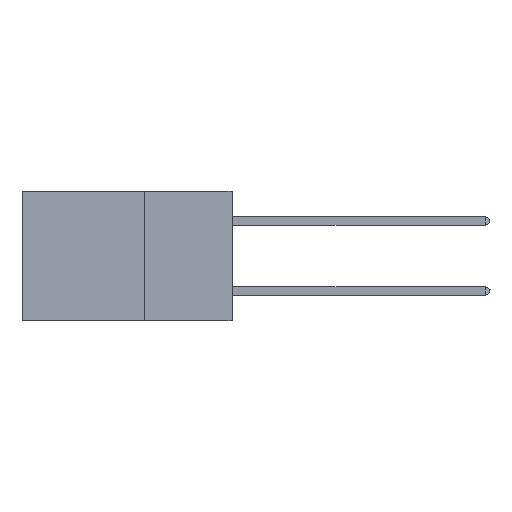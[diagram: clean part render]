
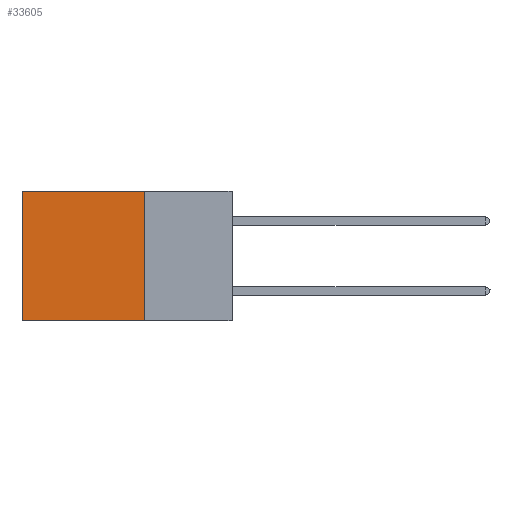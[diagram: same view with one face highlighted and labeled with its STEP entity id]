
A CAD part, left-side view. The second image highlights one B-rep face of the part: STEP entity #33605.
In plain terms, the highlighted planar face has unit normal (-1, 0, 0).
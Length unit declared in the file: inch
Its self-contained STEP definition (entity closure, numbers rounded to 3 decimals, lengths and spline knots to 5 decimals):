
#642 = CARTESIAN_POINT ( 'NONE',  ( 0.2875, 0.6, -0.37 ) ) ;
#1682 = VERTEX_POINT ( 'NONE', #38714 ) ;
#2686 = EDGE_LOOP ( 'NONE', ( #25960, #5199, #11794, #3918 ) ) ;
#3322 = CARTESIAN_POINT ( 'NONE',  ( 0.2875, 0.6, 0. ) ) ;
#3918 = ORIENTED_EDGE ( 'NONE', *, *, #21342, .T. ) ;
#4145 = EDGE_CURVE ( 'NONE', #11083, #21755, #27333, .T. ) ;
#4166 = DIRECTION ( 'NONE',  ( 0., 0., -1. ) ) ;
#5199 = ORIENTED_EDGE ( 'NONE', *, *, #4145, .F. ) ;
#10531 = LINE ( 'NONE', #3322, #20879 ) ;
#11083 = VERTEX_POINT ( 'NONE', #28996 ) ;
#11794 = ORIENTED_EDGE ( 'NONE', *, *, #13632, .F. ) ;
#12346 = DIRECTION ( 'NONE',  ( 0., 1., 0. ) ) ;
#13632 = EDGE_CURVE ( 'NONE', #14306, #11083, #15678, .T. ) ;
#14306 = VERTEX_POINT ( 'NONE', #22664 ) ;
#15541 = VECTOR ( 'NONE', #12346, 39.37008 ) ;
#15678 = LINE ( 'NONE', #35035, #25415 ) ;
#16436 = FACE_OUTER_BOUND ( 'NONE', #2686, .T. ) ;
#20013 = LINE ( 'NONE', #41479, #25109 ) ;
#20447 = PLANE ( 'NONE',  #23503 ) ;
#20879 = VECTOR ( 'NONE', #36404, 39.37008 ) ;
#21342 = EDGE_CURVE ( 'NONE', #14306, #1682, #20013, .T. ) ;
#21755 = VERTEX_POINT ( 'NONE', #642 ) ;
#21946 = DIRECTION ( 'NONE',  ( 0., 1., 0. ) ) ;
#22664 = CARTESIAN_POINT ( 'NONE',  ( 0.2875, 0.25, 0. ) ) ;
#23503 = AXIS2_PLACEMENT_3D ( 'NONE', #23714, #40109, #4166 ) ;
#23714 = CARTESIAN_POINT ( 'NONE',  ( 0.2875, 0.25, 0. ) ) ;
#25109 = VECTOR ( 'NONE', #21946, 39.37008 ) ;
#25415 = VECTOR ( 'NONE', #28753, 39.37008 ) ;
#25960 = ORIENTED_EDGE ( 'NONE', *, *, #38788, .T. ) ;
#27333 = LINE ( 'NONE', #31802, #15541 ) ;
#28753 = DIRECTION ( 'NONE',  ( 0., 0., -1. ) ) ;
#28996 = CARTESIAN_POINT ( 'NONE',  ( 0.2875, 0.25, -0.37 ) ) ;
#31802 = CARTESIAN_POINT ( 'NONE',  ( 0.2875, 0.25, -0.37 ) ) ;
#33605 = ADVANCED_FACE ( 'NONE', ( #16436 ), #20447, .F. ) ;
#35035 = CARTESIAN_POINT ( 'NONE',  ( 0.2875, 0.25, 0. ) ) ;
#36404 = DIRECTION ( 'NONE',  ( 0., 0., -1. ) ) ;
#38714 = CARTESIAN_POINT ( 'NONE',  ( 0.2875, 0.6, 0. ) ) ;
#38788 = EDGE_CURVE ( 'NONE', #1682, #21755, #10531, .T. ) ;
#40109 = DIRECTION ( 'NONE',  ( 1., 0., 0. ) ) ;
#41479 = CARTESIAN_POINT ( 'NONE',  ( 0.2875, 0.25, 0. ) ) ;
